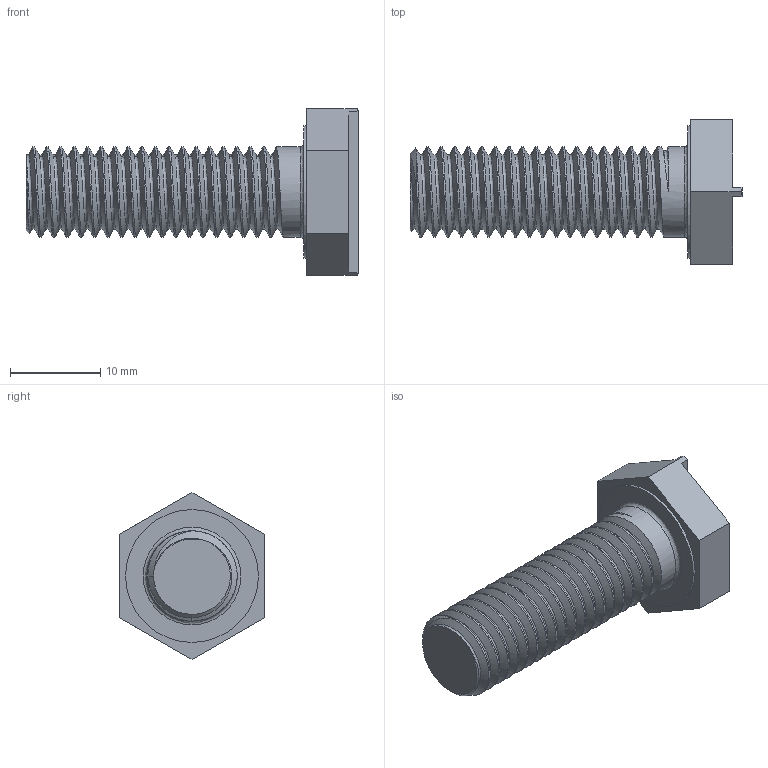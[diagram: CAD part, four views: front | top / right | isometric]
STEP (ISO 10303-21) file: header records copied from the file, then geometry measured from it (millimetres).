
FILE_DESCRIPTION(('FreeCAD Model'),'2;1');
FILE_NAME('Open CASCADE Shape Model','2022-12-07T11:21:54',('Author'),( ''),'Open CASCADE STEP processor 7.6','FreeCAD','Unknown');
FILE_SCHEMA(('AUTOMOTIVE_DESIGN { 1 0 10303 214 1 1 1 1 }'));
Length unit declared in the file: millimetre
Products named in the file (1): M10x30 Breach Face
Bounding box: 36.75 x 16 x 18.48 mm (x, y, z)
Volume: 3133.1 mm3; surface area: 2154.9 mm2
Topology: 1 solids, 1 shells, 100 faces, 249 edges, 153 vertices
Faces by surface type: bspline 60, cylinder 20, plane 14, cone 5, revolution 1
Full cylindrical faces by diameter (mm): 10 x18, 14.7 x1
Entity records: 19535 total; most frequent: CARTESIAN_POINT 15645, ORIENTED_EDGE 498, PCURVE 498, DEFINITIONAL_REPRESENTATION 498, B_SPLINE_CURVE_WITH_KNOTS 455, DIRECTION 345, EDGE_CURVE 249, SURFACE_CURVE 246
